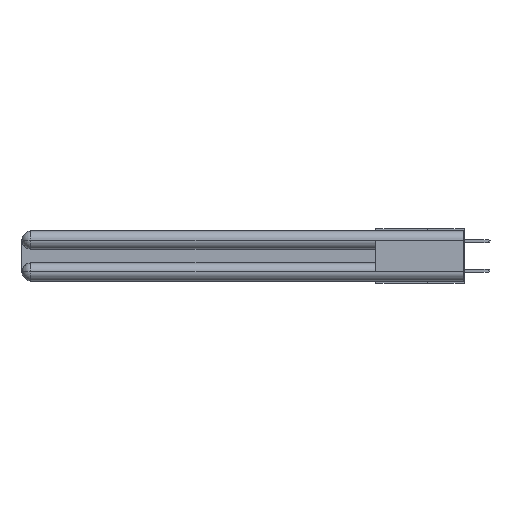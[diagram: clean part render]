
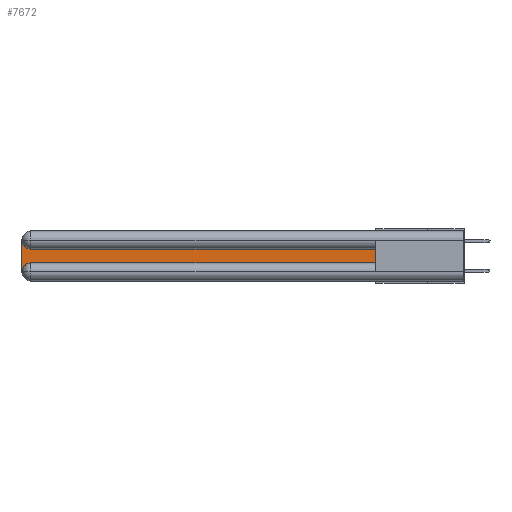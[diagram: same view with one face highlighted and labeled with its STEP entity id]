
A CAD part, left-side view. The second image highlights one B-rep face of the part: STEP entity #7672.
In plain terms, the highlighted planar face has unit normal (-1, 0, 0).
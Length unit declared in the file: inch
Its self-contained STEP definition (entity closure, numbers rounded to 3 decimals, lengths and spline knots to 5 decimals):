
#11 = EDGE_CURVE ( 'NONE', #15338, #6938, #9070, .T. ) ;
#23 = ORIENTED_EDGE ( 'NONE', *, *, #21800, .T. ) ;
#2185 = ORIENTED_EDGE ( 'NONE', *, *, #4471, .T. ) ;
#3746 = LINE ( 'NONE', #22275, #4698 ) ;
#3884 = DIRECTION ( 'NONE',  ( 0., 0., 1. ) ) ;
#3947 = ORIENTED_EDGE ( 'NONE', *, *, #9468, .T. ) ;
#4100 = VERTEX_POINT ( 'NONE', #24752 ) ;
#4471 = EDGE_CURVE ( 'NONE', #5909, #23636, #3746, .T. ) ;
#4698 = VECTOR ( 'NONE', #3884, 39.37008 ) ;
#5443 = DIRECTION ( 'NONE',  ( 1., 0., 0. ) ) ;
#5611 = CARTESIAN_POINT ( 'NONE',  ( 0.075, 2.94, -0.0625 ) ) ;
#5909 = VERTEX_POINT ( 'NONE', #21272 ) ;
#6938 = VERTEX_POINT ( 'NONE', #8972 ) ;
#7147 = DIRECTION ( 'NONE',  ( 1., 0., 0. ) ) ;
#7658 = EDGE_LOOP ( 'NONE', ( #22900, #21431, #23, #3947, #15418, #2185 ) ) ;
#7672 = ADVANCED_FACE ( 'NONE', ( #18861 ), #25918, .F. ) ;
#7708 = CARTESIAN_POINT ( 'NONE',  ( 0.075, 3., -0.2775 ) ) ;
#8972 = CARTESIAN_POINT ( 'NONE',  ( 0.075, 3., -0.0625 ) ) ;
#9005 = DIRECTION ( 'NONE',  ( 0., 1., 0. ) ) ;
#9070 = CIRCLE ( 'NONE', #26398, 0.06 ) ;
#9311 = VECTOR ( 'NONE', #11948, 39.37008 ) ;
#9468 = EDGE_CURVE ( 'NONE', #14773, #4100, #24239, .T. ) ;
#9780 = CARTESIAN_POINT ( 'NONE',  ( 0.075, 0.6, -0.2175 ) ) ;
#10703 = VECTOR ( 'NONE', #19893, 39.37008 ) ;
#10732 = LINE ( 'NONE', #23231, #13354 ) ;
#11948 = DIRECTION ( 'NONE',  ( 0., -1., 0. ) ) ;
#13354 = VECTOR ( 'NONE', #9005, 39.37008 ) ;
#13639 = DIRECTION ( 'NONE',  ( 0., 0., -1. ) ) ;
#13694 = CARTESIAN_POINT ( 'NONE',  ( 0.075, 3., -0.2175 ) ) ;
#14138 = DIRECTION ( 'NONE',  ( 0., 0., -1. ) ) ;
#14773 = VERTEX_POINT ( 'NONE', #7708 ) ;
#14886 = LINE ( 'NONE', #9780, #9311 ) ;
#15338 = VERTEX_POINT ( 'NONE', #26103 ) ;
#15418 = ORIENTED_EDGE ( 'NONE', *, *, #23052, .T. ) ;
#17792 = DIRECTION ( 'NONE',  ( 1., 0., 0. ) ) ;
#18861 = FACE_OUTER_BOUND ( 'NONE', #7658, .T. ) ;
#19661 = CARTESIAN_POINT ( 'NONE',  ( 0.075, 3., -0.1225 ) ) ;
#19893 = DIRECTION ( 'NONE',  ( 0., 0., -1. ) ) ;
#19902 = AXIS2_PLACEMENT_3D ( 'NONE', #26328, #5443, #14138 ) ;
#21272 = CARTESIAN_POINT ( 'NONE',  ( 0.075, 0.6, -0.2175 ) ) ;
#21431 = ORIENTED_EDGE ( 'NONE', *, *, #11, .T. ) ;
#21485 = EDGE_CURVE ( 'NONE', #23636, #15338, #10732, .T. ) ;
#21578 = CARTESIAN_POINT ( 'NONE',  ( 0.075, 0.6, -0.1225 ) ) ;
#21800 = EDGE_CURVE ( 'NONE', #6938, #14773, #26600, .T. ) ;
#22275 = CARTESIAN_POINT ( 'NONE',  ( 0.075, 0.6, -0.2175 ) ) ;
#22900 = ORIENTED_EDGE ( 'NONE', *, *, #21485, .T. ) ;
#23052 = EDGE_CURVE ( 'NONE', #4100, #5909, #14886, .T. ) ;
#23231 = CARTESIAN_POINT ( 'NONE',  ( 0.075, 0.6, -0.1225 ) ) ;
#23636 = VERTEX_POINT ( 'NONE', #21578 ) ;
#24239 = CIRCLE ( 'NONE', #19902, 0.06 ) ;
#24286 = DIRECTION ( 'NONE',  ( 0., 0., -1. ) ) ;
#24752 = CARTESIAN_POINT ( 'NONE',  ( 0.075, 2.94, -0.2175 ) ) ;
#25918 = PLANE ( 'NONE',  #26312 ) ;
#26103 = CARTESIAN_POINT ( 'NONE',  ( 0.075, 2.94, -0.1225 ) ) ;
#26312 = AXIS2_PLACEMENT_3D ( 'NONE', #19661, #7147, #13639 ) ;
#26328 = CARTESIAN_POINT ( 'NONE',  ( 0.075, 2.94, -0.2775 ) ) ;
#26398 = AXIS2_PLACEMENT_3D ( 'NONE', #5611, #17792, #24286 ) ;
#26600 = LINE ( 'NONE', #13694, #10703 ) ;
